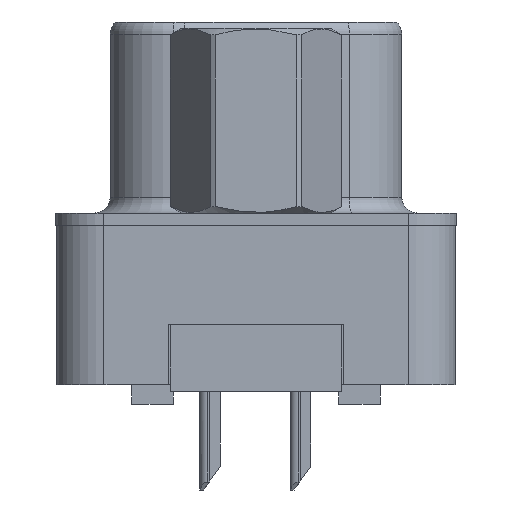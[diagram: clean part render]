
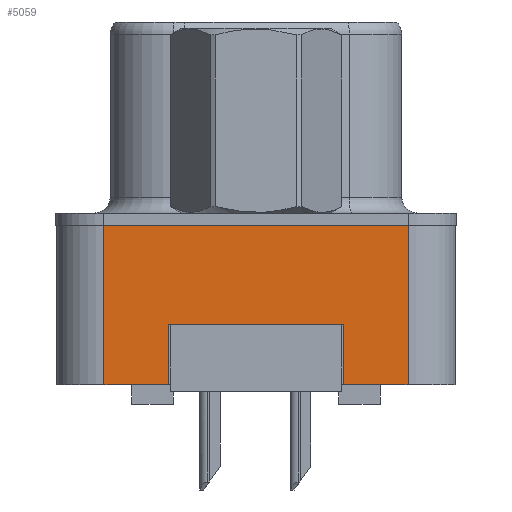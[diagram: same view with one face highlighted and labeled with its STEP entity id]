
A CAD part, left-side view. The second image highlights one B-rep face of the part: STEP entity #5059.
In plain terms, the highlighted planar face has unit normal (-1, 0, 0).
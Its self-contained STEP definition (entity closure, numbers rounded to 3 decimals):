
#814 = VERTEX_POINT ( 'NONE', #19805 ) ;
#837 = LINE ( 'NONE', #11577, #25631 ) ;
#1635 = EDGE_CURVE ( 'NONE', #4790, #12412, #23436, .T. ) ;
#1784 = VECTOR ( 'NONE', #1856, 1000. ) ;
#1856 = DIRECTION ( 'NONE',  ( 0., -1., 0. ) ) ;
#1896 = CARTESIAN_POINT ( 'NONE',  ( -3., -4.775, -5. ) ) ;
#2309 = VERTEX_POINT ( 'NONE', #21947 ) ;
#2845 = CARTESIAN_POINT ( 'NONE',  ( -3., -2.75, -5. ) ) ;
#3660 = DIRECTION ( 'NONE',  ( 0., -1., 0. ) ) ;
#4246 = DIRECTION ( 'NONE',  ( 0., 0., -1. ) ) ;
#4790 = VERTEX_POINT ( 'NONE', #20793 ) ;
#4948 = VECTOR ( 'NONE', #4246, 1000. ) ;
#5059 = ADVANCED_FACE ( 'NONE', ( #12184 ), #18933, .T. ) ;
#5132 = CARTESIAN_POINT ( 'NONE',  ( -3., -4.775, -5. ) ) ;
#5244 = CARTESIAN_POINT ( 'NONE',  ( -3., 4.775, -5. ) ) ;
#5537 = ORIENTED_EDGE ( 'NONE', *, *, #1635, .F. ) ;
#5803 = CARTESIAN_POINT ( 'NONE',  ( -3., -4.775, 0. ) ) ;
#6199 = LINE ( 'NONE', #1896, #23521 ) ;
#7896 = ORIENTED_EDGE ( 'NONE', *, *, #25534, .F. ) ;
#8819 = LINE ( 'NONE', #23872, #4948 ) ;
#9099 = CARTESIAN_POINT ( 'NONE',  ( -3., 4.775, -5. ) ) ;
#9626 = VECTOR ( 'NONE', #26920, 1000. ) ;
#9707 = LINE ( 'NONE', #5132, #9626 ) ;
#9780 = EDGE_CURVE ( 'NONE', #19297, #12412, #6199, .T. ) ;
#10346 = CARTESIAN_POINT ( 'NONE',  ( -3., 2.75, -3.1 ) ) ;
#10909 = DIRECTION ( 'NONE',  ( 0., 0., 1. ) ) ;
#11577 = CARTESIAN_POINT ( 'NONE',  ( -3., 2.75, -3.1 ) ) ;
#12184 = FACE_OUTER_BOUND ( 'NONE', #19900, .T. ) ;
#12412 = VERTEX_POINT ( 'NONE', #26021 ) ;
#12461 = ORIENTED_EDGE ( 'NONE', *, *, #27945, .F. ) ;
#14468 = DIRECTION ( 'NONE',  ( 0., 0., 1. ) ) ;
#14596 = LINE ( 'NONE', #19055, #1784 ) ;
#14658 = ORIENTED_EDGE ( 'NONE', *, *, #23893, .T. ) ;
#14751 = VECTOR ( 'NONE', #25595, 1000. ) ;
#16123 = LINE ( 'NONE', #5244, #20704 ) ;
#16624 = CARTESIAN_POINT ( 'NONE',  ( -3., -4.775, -5. ) ) ;
#16736 = VECTOR ( 'NONE', #3660, 1000. ) ;
#18485 = ORIENTED_EDGE ( 'NONE', *, *, #23031, .T. ) ;
#18933 = PLANE ( 'NONE',  #28000 ) ;
#18966 = ORIENTED_EDGE ( 'NONE', *, *, #9780, .T. ) ;
#19055 = CARTESIAN_POINT ( 'NONE',  ( -3., -4.775, -5. ) ) ;
#19297 = VERTEX_POINT ( 'NONE', #24594 ) ;
#19426 = CARTESIAN_POINT ( 'NONE',  ( -3., 2.75, -3.1 ) ) ;
#19805 = CARTESIAN_POINT ( 'NONE',  ( -3., 2.75, -5. ) ) ;
#19900 = EDGE_LOOP ( 'NONE', ( #18485, #27350, #18966, #5537, #27763, #14658, #7896, #12461 ) ) ;
#20704 = VECTOR ( 'NONE', #23443, 1000. ) ;
#20793 = CARTESIAN_POINT ( 'NONE',  ( -3., 4.775, 0. ) ) ;
#21947 = CARTESIAN_POINT ( 'NONE',  ( -3., -2.75, -3.1 ) ) ;
#23031 = EDGE_CURVE ( 'NONE', #2309, #26025, #8819, .T. ) ;
#23436 = LINE ( 'NONE', #5803, #16736 ) ;
#23443 = DIRECTION ( 'NONE',  ( 0., 0., 1. ) ) ;
#23521 = VECTOR ( 'NONE', #10909, 1000. ) ;
#23872 = CARTESIAN_POINT ( 'NONE',  ( -3., -2.75, -3.1 ) ) ;
#23893 = EDGE_CURVE ( 'NONE', #25896, #814, #14596, .T. ) ;
#24594 = CARTESIAN_POINT ( 'NONE',  ( -3., -4.775, -5. ) ) ;
#24903 = DIRECTION ( 'NONE',  ( 0., 0., -1. ) ) ;
#25312 = VERTEX_POINT ( 'NONE', #10346 ) ;
#25375 = DIRECTION ( 'NONE',  ( -1., 0., 0. ) ) ;
#25534 = EDGE_CURVE ( 'NONE', #25312, #814, #837, .T. ) ;
#25595 = DIRECTION ( 'NONE',  ( 0., 1., 0. ) ) ;
#25631 = VECTOR ( 'NONE', #24903, 1000. ) ;
#25650 = EDGE_CURVE ( 'NONE', #26025, #19297, #9707, .T. ) ;
#25741 = LINE ( 'NONE', #19426, #14751 ) ;
#25896 = VERTEX_POINT ( 'NONE', #9099 ) ;
#26021 = CARTESIAN_POINT ( 'NONE',  ( -3., -4.775, 0. ) ) ;
#26025 = VERTEX_POINT ( 'NONE', #2845 ) ;
#26920 = DIRECTION ( 'NONE',  ( 0., -1., 0. ) ) ;
#27350 = ORIENTED_EDGE ( 'NONE', *, *, #25650, .T. ) ;
#27763 = ORIENTED_EDGE ( 'NONE', *, *, #27916, .F. ) ;
#27916 = EDGE_CURVE ( 'NONE', #25896, #4790, #16123, .T. ) ;
#27945 = EDGE_CURVE ( 'NONE', #2309, #25312, #25741, .T. ) ;
#28000 = AXIS2_PLACEMENT_3D ( 'NONE', #16624, #25375, #14468 ) ;
